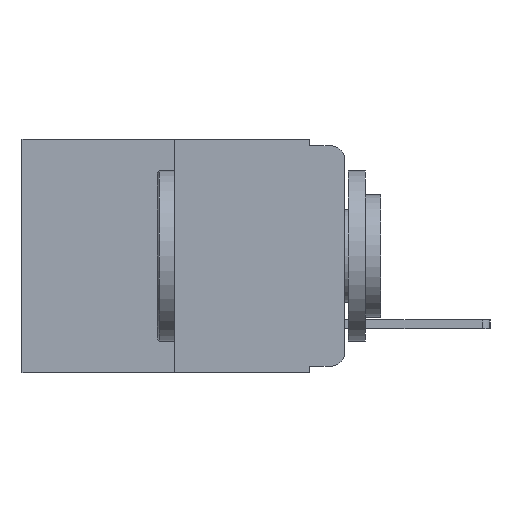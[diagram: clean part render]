
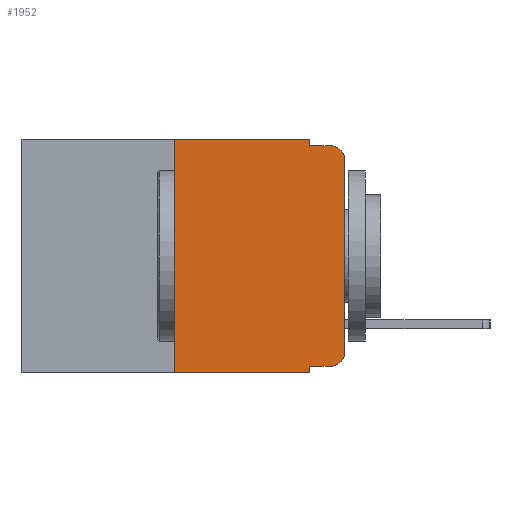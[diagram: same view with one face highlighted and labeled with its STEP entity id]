
A CAD part, left-side view. The second image highlights one B-rep face of the part: STEP entity #1952.
In plain terms, the highlighted planar face has unit normal (-1, 0, 0).
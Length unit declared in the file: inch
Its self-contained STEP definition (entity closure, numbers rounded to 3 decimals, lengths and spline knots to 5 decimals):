
#10 = DIRECTION ( 'NONE',  ( 0., 0., -1. ) ) ;
#115 = LINE ( 'NONE', #8071, #7550 ) ;
#152 = ORIENTED_EDGE ( 'NONE', *, *, #10163, .T. ) ;
#187 = VECTOR ( 'NONE', #9567, 39.37008 ) ;
#311 = DIRECTION ( 'NONE',  ( 0., -1., 0. ) ) ;
#524 = DIRECTION ( 'NONE',  ( 0., -1., 0. ) ) ;
#684 = CARTESIAN_POINT ( 'NONE',  ( 0., 0.051, 0. ) ) ;
#743 = ORIENTED_EDGE ( 'NONE', *, *, #856, .F. ) ;
#752 = CIRCLE ( 'NONE', #10987, 0.02 ) ;
#832 = VERTEX_POINT ( 'NONE', #2437 ) ;
#856 = EDGE_CURVE ( 'NONE', #832, #8834, #2764, .T. ) ;
#949 = DIRECTION ( 'NONE',  ( 0., -1., 0. ) ) ;
#1027 = DIRECTION ( 'NONE',  ( 0., 0., -1. ) ) ;
#1028 = EDGE_LOOP ( 'NONE', ( #2224, #7820, #6037, #743, #8000, #9651, #152, #7731, #6194, #5958 ) ) ;
#1103 = DIRECTION ( 'NONE',  ( 1., 0., 0. ) ) ;
#1296 = PLANE ( 'NONE',  #5161 ) ;
#1797 = CARTESIAN_POINT ( 'NONE',  ( 0., 0.051, -0.01 ) ) ;
#1952 = ADVANCED_FACE ( 'NONE', ( #10238 ), #1296, .F. ) ;
#2148 = DIRECTION ( 'NONE',  ( 0., 0., -1. ) ) ;
#2166 = EDGE_CURVE ( 'NONE', #8834, #11900, #3054, .T. ) ;
#2224 = ORIENTED_EDGE ( 'NONE', *, *, #7378, .T. ) ;
#2232 = VERTEX_POINT ( 'NONE', #4720 ) ;
#2437 = CARTESIAN_POINT ( 'NONE',  ( 0., 0.051, 0. ) ) ;
#2764 = LINE ( 'NONE', #684, #187 ) ;
#2848 = EDGE_CURVE ( 'NONE', #2232, #10217, #752, .T. ) ;
#3054 = LINE ( 'NONE', #1797, #7896 ) ;
#3832 = DIRECTION ( 'NONE',  ( 0., 0., 1. ) ) ;
#3876 = CARTESIAN_POINT ( 'NONE',  ( 0., 0.25, -0.343 ) ) ;
#4144 = CARTESIAN_POINT ( 'NONE',  ( 0., 0.051, 0. ) ) ;
#4386 = LINE ( 'NONE', #4144, #6926 ) ;
#4487 = VECTOR ( 'NONE', #4714, 39.37008 ) ;
#4714 = DIRECTION ( 'NONE',  ( 0., 0., 1. ) ) ;
#4720 = CARTESIAN_POINT ( 'NONE',  ( 0., 0.02, -0.333 ) ) ;
#4889 = CARTESIAN_POINT ( 'NONE',  ( 0., 0.051, -0.333 ) ) ;
#5161 = AXIS2_PLACEMENT_3D ( 'NONE', #12216, #1103, #1027 ) ;
#5835 = DIRECTION ( 'NONE',  ( -1., 0., 0. ) ) ;
#5958 = ORIENTED_EDGE ( 'NONE', *, *, #2848, .T. ) ;
#6037 = ORIENTED_EDGE ( 'NONE', *, *, #2166, .F. ) ;
#6108 = EDGE_CURVE ( 'NONE', #7245, #11900, #10149, .T. ) ;
#6119 = EDGE_CURVE ( 'NONE', #11647, #2232, #12285, .T. ) ;
#6194 = ORIENTED_EDGE ( 'NONE', *, *, #6119, .T. ) ;
#6283 = LINE ( 'NONE', #6728, #11262 ) ;
#6622 = CARTESIAN_POINT ( 'NONE',  ( 0., 0.25, 0. ) ) ;
#6662 = DIRECTION ( 'NONE',  ( 0., -1., 0. ) ) ;
#6723 = LINE ( 'NONE', #10414, #9254 ) ;
#6728 = CARTESIAN_POINT ( 'NONE',  ( 0., 0., 0. ) ) ;
#6926 = VECTOR ( 'NONE', #2148, 39.37008 ) ;
#6939 = VERTEX_POINT ( 'NONE', #10954 ) ;
#7245 = VERTEX_POINT ( 'NONE', #7404 ) ;
#7378 = EDGE_CURVE ( 'NONE', #10217, #7245, #6283, .T. ) ;
#7404 = CARTESIAN_POINT ( 'NONE',  ( 0., 0., -0.03 ) ) ;
#7406 = VERTEX_POINT ( 'NONE', #3876 ) ;
#7550 = VECTOR ( 'NONE', #311, 39.37008 ) ;
#7731 = ORIENTED_EDGE ( 'NONE', *, *, #8257, .F. ) ;
#7765 = CARTESIAN_POINT ( 'NONE',  ( 0., 0.02, -0.313 ) ) ;
#7820 = ORIENTED_EDGE ( 'NONE', *, *, #6108, .T. ) ;
#7896 = VECTOR ( 'NONE', #524, 39.37008 ) ;
#8000 = ORIENTED_EDGE ( 'NONE', *, *, #11998, .F. ) ;
#8071 = CARTESIAN_POINT ( 'NONE',  ( 0., 0.473, 0. ) ) ;
#8228 = DIRECTION ( 'NONE',  ( -1., 0., 0. ) ) ;
#8257 = EDGE_CURVE ( 'NONE', #11647, #6939, #4386, .T. ) ;
#8370 = AXIS2_PLACEMENT_3D ( 'NONE', #11445, #5835, #10 ) ;
#8491 = CARTESIAN_POINT ( 'NONE',  ( 0., 0.051, -0.01 ) ) ;
#8834 = VERTEX_POINT ( 'NONE', #8491 ) ;
#9254 = VECTOR ( 'NONE', #6662, 39.37008 ) ;
#9475 = CARTESIAN_POINT ( 'NONE',  ( 0., 0.051, -0.333 ) ) ;
#9567 = DIRECTION ( 'NONE',  ( 0., 0., -1. ) ) ;
#9610 = CARTESIAN_POINT ( 'NONE',  ( 0., 0., -0.313 ) ) ;
#9651 = ORIENTED_EDGE ( 'NONE', *, *, #10140, .F. ) ;
#9870 = VECTOR ( 'NONE', #949, 39.37008 ) ;
#10140 = EDGE_CURVE ( 'NONE', #7406, #10963, #11679, .T. ) ;
#10149 = CIRCLE ( 'NONE', #8370, 0.02 ) ;
#10163 = EDGE_CURVE ( 'NONE', #7406, #6939, #6723, .T. ) ;
#10217 = VERTEX_POINT ( 'NONE', #9610 ) ;
#10238 = FACE_OUTER_BOUND ( 'NONE', #1028, .T. ) ;
#10414 = CARTESIAN_POINT ( 'NONE',  ( 0., 0.473, -0.343 ) ) ;
#10737 = CARTESIAN_POINT ( 'NONE',  ( 0., 0.02, -0.01 ) ) ;
#10758 = CARTESIAN_POINT ( 'NONE',  ( 0., 0.25, 0. ) ) ;
#10954 = CARTESIAN_POINT ( 'NONE',  ( 0., 0.051, -0.343 ) ) ;
#10963 = VERTEX_POINT ( 'NONE', #10758 ) ;
#10987 = AXIS2_PLACEMENT_3D ( 'NONE', #7765, #8228, #11378 ) ;
#11262 = VECTOR ( 'NONE', #3832, 39.37008 ) ;
#11378 = DIRECTION ( 'NONE',  ( 0., 0., -1. ) ) ;
#11445 = CARTESIAN_POINT ( 'NONE',  ( 0., 0.02, -0.03 ) ) ;
#11647 = VERTEX_POINT ( 'NONE', #9475 ) ;
#11679 = LINE ( 'NONE', #6622, #4487 ) ;
#11900 = VERTEX_POINT ( 'NONE', #10737 ) ;
#11998 = EDGE_CURVE ( 'NONE', #10963, #832, #115, .T. ) ;
#12216 = CARTESIAN_POINT ( 'NONE',  ( 0., 0.473, 0. ) ) ;
#12285 = LINE ( 'NONE', #4889, #9870 ) ;
